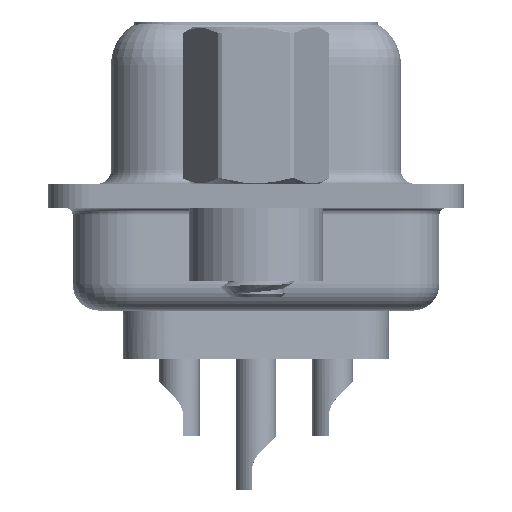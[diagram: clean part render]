
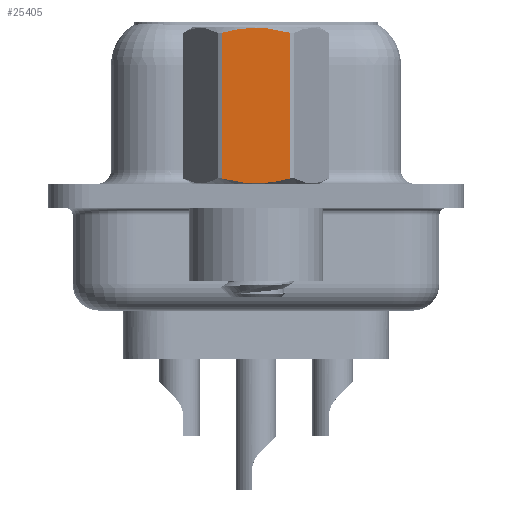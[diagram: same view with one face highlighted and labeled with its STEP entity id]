
A CAD part, left-side view. The second image highlights one B-rep face of the part: STEP entity #25405.
In plain terms, the highlighted planar face has unit normal (-1, 0, 0).
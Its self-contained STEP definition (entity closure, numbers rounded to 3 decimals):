
#2270 = VERTEX_POINT ( 'NONE', #13159 ) ;
#2349 = CARTESIAN_POINT ( 'NONE',  ( -2.381, 0.215, 0.468 ) ) ;
#4031 = EDGE_LOOP ( 'NONE', ( #21160, #33582, #29150, #36979 ) ) ;
#4325 = CARTESIAN_POINT ( 'NONE',  ( -2.381, -0.858, 6.15 ) ) ;
#4819 = CARTESIAN_POINT ( 'NONE',  ( -2.381, -1.273, 3.792 ) ) ;
#5656 = CARTESIAN_POINT ( 'NONE',  ( -2.381, -0.432, 0.485 ) ) ;
#6692 = VECTOR ( 'NONE', #21822, 1000. ) ;
#7076 = CARTESIAN_POINT ( 'NONE',  ( -2.381, 1.375, -3.75 ) ) ;
#7581 = CARTESIAN_POINT ( 'NONE',  ( -2.381, -0.215, 6.232 ) ) ;
#8940 = CARTESIAN_POINT ( 'NONE',  ( -2.381, -1.066, 0.596 ) ) ;
#9642 = CARTESIAN_POINT ( 'NONE',  ( -2.381, -1.273, 0.652 ) ) ;
#10114 = EDGE_CURVE ( 'NONE', #2270, #39378, #19357, .T. ) ;
#10369 = DIRECTION ( 'NONE',  ( 0., -1., 0. ) ) ;
#10909 = CARTESIAN_POINT ( 'NONE',  ( -2.381, 0.428, 6.215 ) ) ;
#10958 = VECTOR ( 'NONE', #27955, 1000. ) ;
#13113 = CARTESIAN_POINT ( 'NONE',  ( -2.381, 1.273, 6.048 ) ) ;
#13159 = CARTESIAN_POINT ( 'NONE',  ( -2.381, 1.273, 0.652 ) ) ;
#14114 = CARTESIAN_POINT ( 'NONE',  ( -2.381, -1.273, 6.048 ) ) ;
#14259 = CARTESIAN_POINT ( 'NONE',  ( -2.381, 1.065, 6.104 ) ) ;
#14447 = EDGE_CURVE ( 'NONE', #39378, #37387, #37261, .T. ) ;
#15478 = CARTESIAN_POINT ( 'NONE',  ( -2.381, 1.065, 0.596 ) ) ;
#17445 = CARTESIAN_POINT ( 'NONE',  ( -2.381, -1.066, 6.104 ) ) ;
#18102 = EDGE_CURVE ( 'NONE', #25988, #2270, #33036, .T. ) ;
#19357 = B_SPLINE_CURVE_WITH_KNOTS ( 'NONE', 3,
 ( #38464, #15478, #41882, #22083, #2349, #25470, #5656, #28796, #8940, #32055 ),
 .UNSPECIFIED., .F., .F.,
 ( 4, 2, 2, 2, 4 ),
 ( 0.003, 0.003, 0.004, 0.004, 0.005 ),
 .UNSPECIFIED. ) ;
#21160 = ORIENTED_EDGE ( 'NONE', *, *, #10114, .T. ) ;
#21822 = DIRECTION ( 'NONE',  ( 0., 0., -1. ) ) ;
#22083 = CARTESIAN_POINT ( 'NONE',  ( -2.381, 0.428, 0.485 ) ) ;
#25405 = ADVANCED_FACE ( 'NONE', ( #30275 ), #26904, .T. ) ;
#25470 = CARTESIAN_POINT ( 'NONE',  ( -2.381, -0.215, 0.468 ) ) ;
#25988 = VERTEX_POINT ( 'NONE', #13113 ) ;
#26904 = PLANE ( 'NONE',  #40688 ) ;
#27447 = CARTESIAN_POINT ( 'NONE',  ( -2.381, -0.432, 6.215 ) ) ;
#27955 = DIRECTION ( 'NONE',  ( 0., 0., 1. ) ) ;
#28186 = EDGE_CURVE ( 'NONE', #37387, #25988, #41352, .T. ) ;
#28796 = CARTESIAN_POINT ( 'NONE',  ( -2.381, -0.858, 0.55 ) ) ;
#29150 = ORIENTED_EDGE ( 'NONE', *, *, #28186, .T. ) ;
#30223 = DIRECTION ( 'NONE',  ( -1., 0., 0. ) ) ;
#30275 = FACE_OUTER_BOUND ( 'NONE', #4031, .T. ) ;
#30743 = CARTESIAN_POINT ( 'NONE',  ( -2.381, 0.215, 6.232 ) ) ;
#32055 = CARTESIAN_POINT ( 'NONE',  ( -2.381, -1.273, 0.652 ) ) ;
#33036 = LINE ( 'NONE', #34957, #6692 ) ;
#33582 = ORIENTED_EDGE ( 'NONE', *, *, #14447, .T. ) ;
#34032 = CARTESIAN_POINT ( 'NONE',  ( -2.381, 0.853, 6.151 ) ) ;
#34957 = CARTESIAN_POINT ( 'NONE',  ( -2.381, 1.273, 3.792 ) ) ;
#36017 = CARTESIAN_POINT ( 'NONE',  ( -2.381, -1.273, 6.048 ) ) ;
#36979 = ORIENTED_EDGE ( 'NONE', *, *, #18102, .T. ) ;
#37261 = LINE ( 'NONE', #4819, #10958 ) ;
#37279 = CARTESIAN_POINT ( 'NONE',  ( -2.381, 1.273, 6.048 ) ) ;
#37387 = VERTEX_POINT ( 'NONE', #36017 ) ;
#38464 = CARTESIAN_POINT ( 'NONE',  ( -2.381, 1.273, 0.652 ) ) ;
#39378 = VERTEX_POINT ( 'NONE', #9642 ) ;
#40688 = AXIS2_PLACEMENT_3D ( 'NONE', #7076, #30223, #10369 ) ;
#41352 = B_SPLINE_CURVE_WITH_KNOTS ( 'NONE', 3,
 ( #14114, #17445, #4325, #27447, #7581, #30743, #10909, #34032, #14259, #37279 ),
 .UNSPECIFIED., .F., .F.,
 ( 4, 2, 2, 2, 4 ),
 ( 0.001, 0.002, 0.002, 0.003, 0.004 ),
 .UNSPECIFIED. ) ;
#41882 = CARTESIAN_POINT ( 'NONE',  ( -2.381, 0.853, 0.549 ) ) ;
